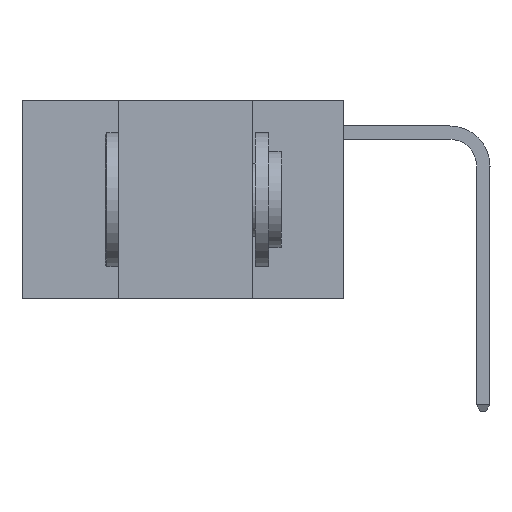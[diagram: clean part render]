
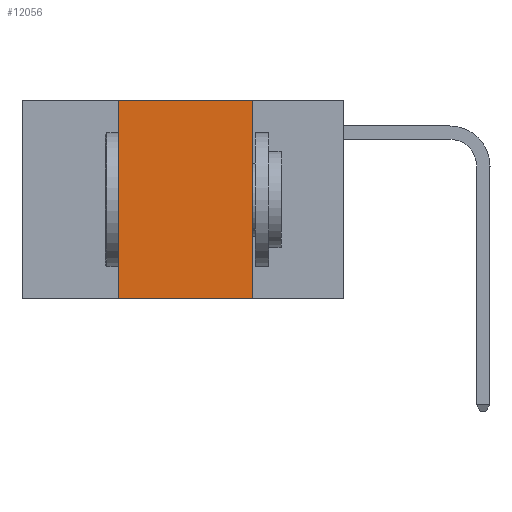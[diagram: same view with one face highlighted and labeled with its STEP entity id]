
A CAD part, left-side view. The second image highlights one B-rep face of the part: STEP entity #12056.
In plain terms, the highlighted planar face has unit normal (-1, 0, 0).
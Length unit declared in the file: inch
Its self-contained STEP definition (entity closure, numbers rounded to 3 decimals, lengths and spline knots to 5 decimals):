
#201 = LINE ( 'NONE', #2323, #5017 ) ;
#534 = EDGE_CURVE ( 'NONE', #4682, #6158, #10654, .T. ) ;
#627 = DIRECTION ( 'NONE',  ( 0., -1., 0. ) ) ;
#739 = EDGE_CURVE ( 'NONE', #2119, #1705, #7549, .T. ) ;
#1106 = DIRECTION ( 'NONE',  ( 1., 0., 0. ) ) ;
#1317 = CARTESIAN_POINT ( 'NONE',  ( 0., 0.17, -0.37 ) ) ;
#1324 = ORIENTED_EDGE ( 'NONE', *, *, #1446, .T. ) ;
#1376 = EDGE_CURVE ( 'NONE', #1705, #4682, #6622, .T. ) ;
#1421 = CARTESIAN_POINT ( 'NONE',  ( 0., 0.17, 0. ) ) ;
#1446 = EDGE_CURVE ( 'NONE', #2119, #6158, #201, .T. ) ;
#1702 = EDGE_LOOP ( 'NONE', ( #6913, #9841, #9858, #1324 ) ) ;
#1705 = VERTEX_POINT ( 'NONE', #10833 ) ;
#2119 = VERTEX_POINT ( 'NONE', #5047 ) ;
#2323 = CARTESIAN_POINT ( 'NONE',  ( 0., 0.6, -0.37 ) ) ;
#3092 = DIRECTION ( 'NONE',  ( 0., -1., 0. ) ) ;
#4682 = VERTEX_POINT ( 'NONE', #1421 ) ;
#5017 = VECTOR ( 'NONE', #627, 39.37008 ) ;
#5047 = CARTESIAN_POINT ( 'NONE',  ( 0., 0.42, -0.37 ) ) ;
#5391 = VECTOR ( 'NONE', #10380, 39.37008 ) ;
#5625 = AXIS2_PLACEMENT_3D ( 'NONE', #11081, #1106, #8173 ) ;
#5813 = DIRECTION ( 'NONE',  ( 0., 0., 1. ) ) ;
#5949 = FACE_OUTER_BOUND ( 'NONE', #1702, .T. ) ;
#5988 = CARTESIAN_POINT ( 'NONE',  ( 0., 0.42, 0. ) ) ;
#6158 = VERTEX_POINT ( 'NONE', #1317 ) ;
#6172 = CARTESIAN_POINT ( 'NONE',  ( 0., 0.6, 0. ) ) ;
#6622 = LINE ( 'NONE', #6172, #9222 ) ;
#6913 = ORIENTED_EDGE ( 'NONE', *, *, #534, .F. ) ;
#7549 = LINE ( 'NONE', #5988, #9554 ) ;
#8173 = DIRECTION ( 'NONE',  ( 0., 0., -1. ) ) ;
#9222 = VECTOR ( 'NONE', #3092, 39.37008 ) ;
#9554 = VECTOR ( 'NONE', #5813, 39.37008 ) ;
#9841 = ORIENTED_EDGE ( 'NONE', *, *, #1376, .F. ) ;
#9858 = ORIENTED_EDGE ( 'NONE', *, *, #739, .F. ) ;
#10138 = PLANE ( 'NONE',  #5625 ) ;
#10380 = DIRECTION ( 'NONE',  ( 0., 0., -1. ) ) ;
#10654 = LINE ( 'NONE', #10715, #5391 ) ;
#10715 = CARTESIAN_POINT ( 'NONE',  ( 0., 0.17, 0. ) ) ;
#10833 = CARTESIAN_POINT ( 'NONE',  ( 0., 0.42, 0. ) ) ;
#11081 = CARTESIAN_POINT ( 'NONE',  ( 0., 0.6, 0. ) ) ;
#12056 = ADVANCED_FACE ( 'NONE', ( #5949 ), #10138, .F. ) ;
